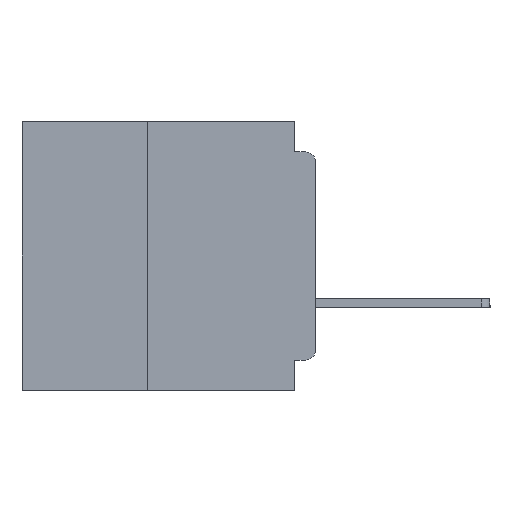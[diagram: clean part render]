
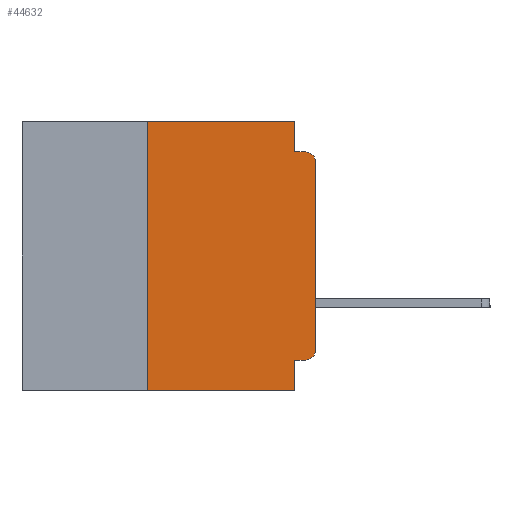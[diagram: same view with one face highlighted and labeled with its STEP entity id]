
A CAD part, left-side view. The second image highlights one B-rep face of the part: STEP entity #44632.
In plain terms, the highlighted planar face has unit normal (-1, 0, 0).
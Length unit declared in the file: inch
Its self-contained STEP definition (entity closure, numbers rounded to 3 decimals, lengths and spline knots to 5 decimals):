
#137 = CARTESIAN_POINT ( 'NONE',  ( 0., 0.031, -0.355 ) ) ;
#289 = VECTOR ( 'NONE', #36376, 39.37008 ) ;
#292 = LINE ( 'NONE', #7877, #43982 ) ;
#802 = DIRECTION ( 'NONE',  ( 0., 0., 1. ) ) ;
#1753 = AXIS2_PLACEMENT_3D ( 'NONE', #19379, #22895, #2052 ) ;
#2052 = DIRECTION ( 'NONE',  ( 0., 0., -1. ) ) ;
#2106 = ORIENTED_EDGE ( 'NONE', *, *, #22101, .T. ) ;
#2551 = CARTESIAN_POINT ( 'NONE',  ( 0., 0.031, 0. ) ) ;
#2696 = VERTEX_POINT ( 'NONE', #35464 ) ;
#3142 = CARTESIAN_POINT ( 'NONE',  ( 0., 0., 0. ) ) ;
#4194 = EDGE_CURVE ( 'NONE', #14987, #32767, #26641, .T. ) ;
#4276 = ORIENTED_EDGE ( 'NONE', *, *, #31020, .F. ) ;
#4589 = LINE ( 'NONE', #20885, #40225 ) ;
#4997 = ORIENTED_EDGE ( 'NONE', *, *, #23003, .F. ) ;
#7099 = DIRECTION ( 'NONE',  ( 0., -1., 0. ) ) ;
#7866 = CARTESIAN_POINT ( 'NONE',  ( 0., 0., -0.34 ) ) ;
#7877 = CARTESIAN_POINT ( 'NONE',  ( 0., 0.25, -0.4 ) ) ;
#9604 = LINE ( 'NONE', #15660, #289 ) ;
#10173 = VECTOR ( 'NONE', #20455, 39.37008 ) ;
#10189 = PLANE ( 'NONE',  #1753 ) ;
#10258 = ORIENTED_EDGE ( 'NONE', *, *, #18021, .F. ) ;
#10270 = CARTESIAN_POINT ( 'NONE',  ( 0., 0.015, -0.045 ) ) ;
#10968 = ORIENTED_EDGE ( 'NONE', *, *, #33597, .F. ) ;
#11012 = VERTEX_POINT ( 'NONE', #137 ) ;
#11494 = ORIENTED_EDGE ( 'NONE', *, *, #15345, .F. ) ;
#12955 = EDGE_LOOP ( 'NONE', ( #14146, #22865, #11494, #10968, #4997, #10258, #30859, #4276, #28748, #2106 ) ) ;
#13782 = CARTESIAN_POINT ( 'NONE',  ( 0., 0., -0.06 ) ) ;
#14146 = ORIENTED_EDGE ( 'NONE', *, *, #17798, .T. ) ;
#14216 = VECTOR ( 'NONE', #41125, 39.37008 ) ;
#14480 = DIRECTION ( 'NONE',  ( -1., 0., 0. ) ) ;
#14692 = LINE ( 'NONE', #43097, #32038 ) ;
#14987 = VERTEX_POINT ( 'NONE', #13782 ) ;
#15345 = EDGE_CURVE ( 'NONE', #16729, #32767, #41642, .T. ) ;
#15660 = CARTESIAN_POINT ( 'NONE',  ( 0., 0.031, 0. ) ) ;
#16368 = LINE ( 'NONE', #37754, #14216 ) ;
#16556 = VECTOR ( 'NONE', #32166, 39.37008 ) ;
#16729 = VERTEX_POINT ( 'NONE', #38315 ) ;
#17640 = LINE ( 'NONE', #32313, #16556 ) ;
#17798 = EDGE_CURVE ( 'NONE', #41916, #14987, #18307, .T. ) ;
#18021 = EDGE_CURVE ( 'NONE', #27335, #37523, #292, .T. ) ;
#18307 = LINE ( 'NONE', #3142, #10173 ) ;
#19146 = DIRECTION ( 'NONE',  ( 0., -1., 0. ) ) ;
#19379 = CARTESIAN_POINT ( 'NONE',  ( 0., 0.437, 0. ) ) ;
#20113 = DIRECTION ( 'NONE',  ( 0., 0., -1. ) ) ;
#20455 = DIRECTION ( 'NONE',  ( 0., 0., 1. ) ) ;
#20494 = DIRECTION ( 'NONE',  ( -1., 0., 0. ) ) ;
#20885 = CARTESIAN_POINT ( 'NONE',  ( 0., 0.437, -0.4 ) ) ;
#21041 = CARTESIAN_POINT ( 'NONE',  ( 0., 0.015, -0.06 ) ) ;
#22101 = EDGE_CURVE ( 'NONE', #39572, #41916, #33203, .T. ) ;
#22865 = ORIENTED_EDGE ( 'NONE', *, *, #4194, .T. ) ;
#22871 = CARTESIAN_POINT ( 'NONE',  ( 0., 0., -0.045 ) ) ;
#22895 = DIRECTION ( 'NONE',  ( 1., 0., 0. ) ) ;
#23003 = EDGE_CURVE ( 'NONE', #37523, #37689, #14692, .T. ) ;
#25880 = EDGE_CURVE ( 'NONE', #39572, #11012, #17640, .T. ) ;
#26361 = DIRECTION ( 'NONE',  ( 0., -1., 0. ) ) ;
#26641 = CIRCLE ( 'NONE', #43696, 0.015 ) ;
#27335 = VERTEX_POINT ( 'NONE', #33981 ) ;
#28748 = ORIENTED_EDGE ( 'NONE', *, *, #25880, .F. ) ;
#28853 = EDGE_CURVE ( 'NONE', #27335, #2696, #4589, .T. ) ;
#30859 = ORIENTED_EDGE ( 'NONE', *, *, #28853, .T. ) ;
#31020 = EDGE_CURVE ( 'NONE', #11012, #2696, #16368, .T. ) ;
#31569 = VECTOR ( 'NONE', #26361, 39.37008 ) ;
#32038 = VECTOR ( 'NONE', #19146, 39.37008 ) ;
#32166 = DIRECTION ( 'NONE',  ( 0., 1., 0. ) ) ;
#32313 = CARTESIAN_POINT ( 'NONE',  ( 0., 0., -0.355 ) ) ;
#32767 = VERTEX_POINT ( 'NONE', #10270 ) ;
#33203 = CIRCLE ( 'NONE', #39763, 0.015 ) ;
#33597 = EDGE_CURVE ( 'NONE', #37689, #16729, #9604, .T. ) ;
#33981 = CARTESIAN_POINT ( 'NONE',  ( 0., 0.25, -0.4 ) ) ;
#35201 = CARTESIAN_POINT ( 'NONE',  ( 0., 0.015, -0.34 ) ) ;
#35464 = CARTESIAN_POINT ( 'NONE',  ( 0., 0.031, -0.4 ) ) ;
#36376 = DIRECTION ( 'NONE',  ( 0., 0., -1. ) ) ;
#37523 = VERTEX_POINT ( 'NONE', #39747 ) ;
#37689 = VERTEX_POINT ( 'NONE', #2551 ) ;
#37754 = CARTESIAN_POINT ( 'NONE',  ( 0., 0.031, -0.4 ) ) ;
#38315 = CARTESIAN_POINT ( 'NONE',  ( 0., 0.031, -0.045 ) ) ;
#38625 = DIRECTION ( 'NONE',  ( 0., 0., -1. ) ) ;
#39572 = VERTEX_POINT ( 'NONE', #41440 ) ;
#39747 = CARTESIAN_POINT ( 'NONE',  ( 0., 0.25, 0. ) ) ;
#39763 = AXIS2_PLACEMENT_3D ( 'NONE', #35201, #14480, #38625 ) ;
#40225 = VECTOR ( 'NONE', #7099, 39.37008 ) ;
#41125 = DIRECTION ( 'NONE',  ( 0., 0., -1. ) ) ;
#41349 = FACE_OUTER_BOUND ( 'NONE', #12955, .T. ) ;
#41440 = CARTESIAN_POINT ( 'NONE',  ( 0., 0.015, -0.355 ) ) ;
#41642 = LINE ( 'NONE', #22871, #31569 ) ;
#41916 = VERTEX_POINT ( 'NONE', #7866 ) ;
#43097 = CARTESIAN_POINT ( 'NONE',  ( 0., 0.437, 0. ) ) ;
#43696 = AXIS2_PLACEMENT_3D ( 'NONE', #21041, #20494, #20113 ) ;
#43982 = VECTOR ( 'NONE', #802, 39.37008 ) ;
#44632 = ADVANCED_FACE ( 'NONE', ( #41349 ), #10189, .F. ) ;
